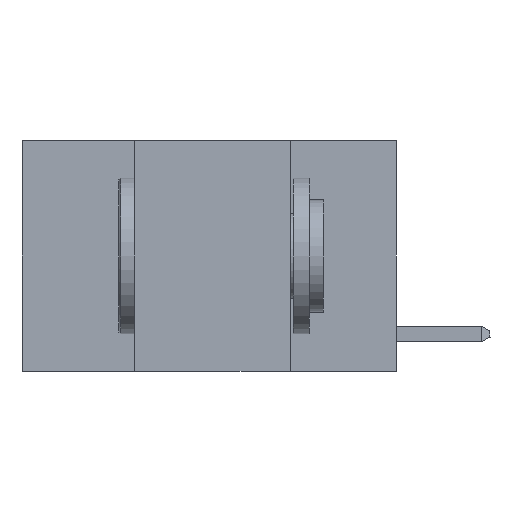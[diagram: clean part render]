
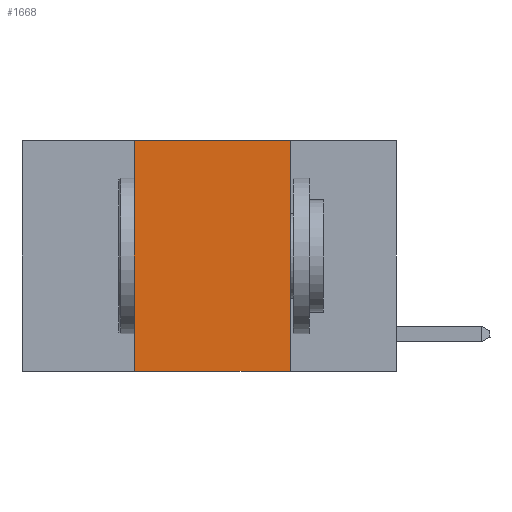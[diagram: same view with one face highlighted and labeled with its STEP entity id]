
A CAD part, left-side view. The second image highlights one B-rep face of the part: STEP entity #1668.
In plain terms, the highlighted planar face has unit normal (-1, 0, 0).
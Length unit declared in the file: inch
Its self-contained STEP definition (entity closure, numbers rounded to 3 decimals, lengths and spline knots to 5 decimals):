
#905 = EDGE_LOOP ( 'NONE', ( #5125, #1374, #7222, #3662 ) ) ;
#1236 = VECTOR ( 'NONE', #5317, 39.37008 ) ;
#1374 = ORIENTED_EDGE ( 'NONE', *, *, #7465, .F. ) ;
#1389 = EDGE_CURVE ( 'NONE', #1657, #6548, #5198, .T. ) ;
#1642 = VECTOR ( 'NONE', #2441, 39.37008 ) ;
#1657 = VERTEX_POINT ( 'NONE', #5600 ) ;
#1668 = ADVANCED_FACE ( 'NONE', ( #5348 ), #6865, .F. ) ;
#1733 = CARTESIAN_POINT ( 'NONE',  ( 0., 0.6, -0.37 ) ) ;
#2052 = AXIS2_PLACEMENT_3D ( 'NONE', #4839, #6451, #5535 ) ;
#2441 = DIRECTION ( 'NONE',  ( 0., -1., 0. ) ) ;
#2614 = CARTESIAN_POINT ( 'NONE',  ( 0., 0.42, 0. ) ) ;
#3579 = EDGE_CURVE ( 'NONE', #6820, #9320, #6431, .T. ) ;
#3662 = ORIENTED_EDGE ( 'NONE', *, *, #8348, .T. ) ;
#3691 = LINE ( 'NONE', #5357, #1642 ) ;
#3799 = CARTESIAN_POINT ( 'NONE',  ( 0., 0.17, 0. ) ) ;
#3852 = VECTOR ( 'NONE', #6881, 39.37008 ) ;
#4057 = CARTESIAN_POINT ( 'NONE',  ( 0., 0.42, 0. ) ) ;
#4111 = DIRECTION ( 'NONE',  ( 0., 0., 1. ) ) ;
#4839 = CARTESIAN_POINT ( 'NONE',  ( 0., 0.6, 0. ) ) ;
#5125 = ORIENTED_EDGE ( 'NONE', *, *, #1389, .F. ) ;
#5198 = LINE ( 'NONE', #3799, #1236 ) ;
#5317 = DIRECTION ( 'NONE',  ( 0., 0., -1. ) ) ;
#5348 = FACE_OUTER_BOUND ( 'NONE', #905, .T. ) ;
#5357 = CARTESIAN_POINT ( 'NONE',  ( 0., 0.6, 0. ) ) ;
#5441 = CARTESIAN_POINT ( 'NONE',  ( 0., 0.17, -0.37 ) ) ;
#5535 = DIRECTION ( 'NONE',  ( 0., 0., -1. ) ) ;
#5600 = CARTESIAN_POINT ( 'NONE',  ( 0., 0.17, 0. ) ) ;
#6431 = LINE ( 'NONE', #4057, #7093 ) ;
#6451 = DIRECTION ( 'NONE',  ( 1., 0., 0. ) ) ;
#6548 = VERTEX_POINT ( 'NONE', #5441 ) ;
#6820 = VERTEX_POINT ( 'NONE', #9108 ) ;
#6865 = PLANE ( 'NONE',  #2052 ) ;
#6881 = DIRECTION ( 'NONE',  ( 0., -1., 0. ) ) ;
#7093 = VECTOR ( 'NONE', #4111, 39.37008 ) ;
#7222 = ORIENTED_EDGE ( 'NONE', *, *, #3579, .F. ) ;
#7465 = EDGE_CURVE ( 'NONE', #9320, #1657, #3691, .T. ) ;
#7613 = LINE ( 'NONE', #1733, #3852 ) ;
#8348 = EDGE_CURVE ( 'NONE', #6820, #6548, #7613, .T. ) ;
#9108 = CARTESIAN_POINT ( 'NONE',  ( 0., 0.42, -0.37 ) ) ;
#9320 = VERTEX_POINT ( 'NONE', #2614 ) ;
